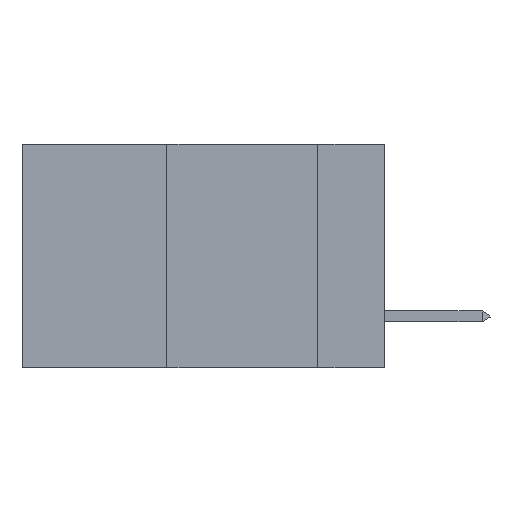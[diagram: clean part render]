
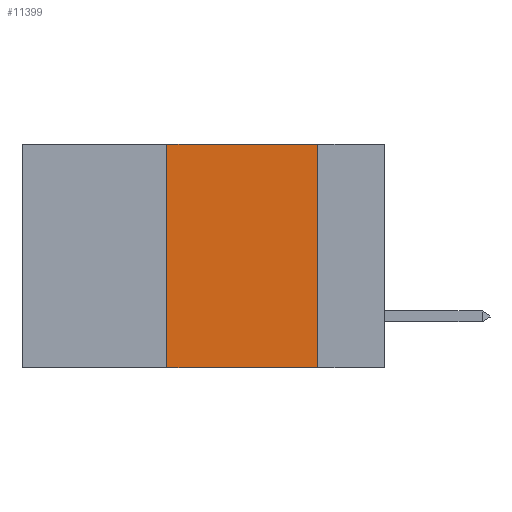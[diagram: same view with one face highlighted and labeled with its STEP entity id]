
A CAD part, left-side view. The second image highlights one B-rep face of the part: STEP entity #11399.
In plain terms, the highlighted planar face has unit normal (-1, 0, 0).
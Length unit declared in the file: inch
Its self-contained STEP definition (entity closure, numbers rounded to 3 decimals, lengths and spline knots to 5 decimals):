
#521 = DIRECTION ( 'NONE',  ( 0., 0., 1. ) ) ;
#1206 = EDGE_CURVE ( 'NONE', #6482, #5399, #6443, .T. ) ;
#1321 = LINE ( 'NONE', #4293, #11318 ) ;
#2674 = CARTESIAN_POINT ( 'NONE',  ( 0., 0.36, 0. ) ) ;
#2758 = VERTEX_POINT ( 'NONE', #3749 ) ;
#3729 = AXIS2_PLACEMENT_3D ( 'NONE', #10289, #7839, #7884 ) ;
#3749 = CARTESIAN_POINT ( 'NONE',  ( 0., 0.11, 0. ) ) ;
#3973 = ORIENTED_EDGE ( 'NONE', *, *, #1206, .F. ) ;
#4193 = CARTESIAN_POINT ( 'NONE',  ( 0., 0.36, 0. ) ) ;
#4242 = EDGE_CURVE ( 'NONE', #2758, #13392, #8525, .T. ) ;
#4293 = CARTESIAN_POINT ( 'NONE',  ( 0., 0.6, -0.37 ) ) ;
#4541 = DIRECTION ( 'NONE',  ( 0., -1., 0. ) ) ;
#5399 = VERTEX_POINT ( 'NONE', #4193 ) ;
#6443 = LINE ( 'NONE', #2674, #14512 ) ;
#6482 = VERTEX_POINT ( 'NONE', #7059 ) ;
#6788 = PLANE ( 'NONE',  #3729 ) ;
#6808 = CARTESIAN_POINT ( 'NONE',  ( 0., 0.11, -0.37 ) ) ;
#6970 = EDGE_LOOP ( 'NONE', ( #7304, #14159, #3973, #7413 ) ) ;
#7059 = CARTESIAN_POINT ( 'NONE',  ( 0., 0.36, -0.37 ) ) ;
#7070 = EDGE_CURVE ( 'NONE', #5399, #2758, #7643, .T. ) ;
#7304 = ORIENTED_EDGE ( 'NONE', *, *, #4242, .F. ) ;
#7413 = ORIENTED_EDGE ( 'NONE', *, *, #10144, .T. ) ;
#7643 = LINE ( 'NONE', #14392, #13274 ) ;
#7839 = DIRECTION ( 'NONE',  ( 1., 0., 0. ) ) ;
#7884 = DIRECTION ( 'NONE',  ( 0., 0., -1. ) ) ;
#8525 = LINE ( 'NONE', #11234, #11865 ) ;
#9986 = DIRECTION ( 'NONE',  ( 0., -1., 0. ) ) ;
#10144 = EDGE_CURVE ( 'NONE', #6482, #13392, #1321, .T. ) ;
#10289 = CARTESIAN_POINT ( 'NONE',  ( 0., 0.6, 0. ) ) ;
#11234 = CARTESIAN_POINT ( 'NONE',  ( 0., 0.11, 0. ) ) ;
#11318 = VECTOR ( 'NONE', #9986, 39.37008 ) ;
#11399 = ADVANCED_FACE ( 'NONE', ( #13189 ), #6788, .F. ) ;
#11865 = VECTOR ( 'NONE', #12177, 39.37008 ) ;
#12177 = DIRECTION ( 'NONE',  ( 0., 0., -1. ) ) ;
#13189 = FACE_OUTER_BOUND ( 'NONE', #6970, .T. ) ;
#13274 = VECTOR ( 'NONE', #4541, 39.37008 ) ;
#13392 = VERTEX_POINT ( 'NONE', #6808 ) ;
#14159 = ORIENTED_EDGE ( 'NONE', *, *, #7070, .F. ) ;
#14392 = CARTESIAN_POINT ( 'NONE',  ( 0., 0.6, 0. ) ) ;
#14512 = VECTOR ( 'NONE', #521, 39.37008 ) ;
